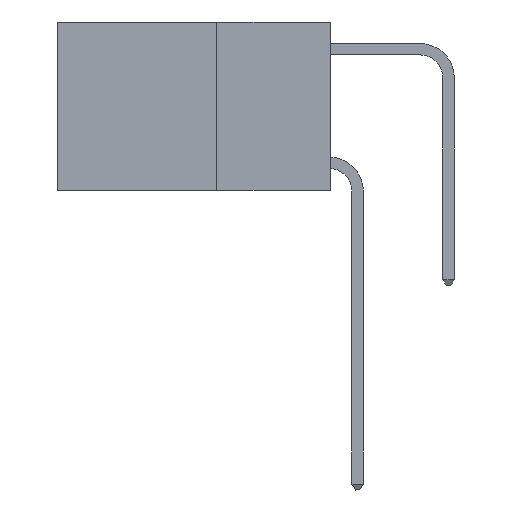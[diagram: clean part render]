
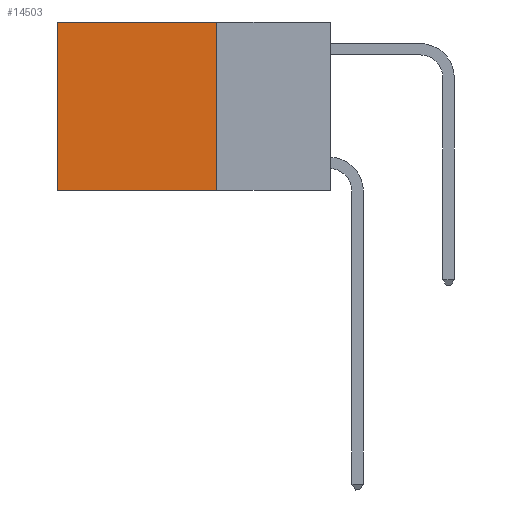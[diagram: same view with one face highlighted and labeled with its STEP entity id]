
A CAD part, left-side view. The second image highlights one B-rep face of the part: STEP entity #14503.
In plain terms, the highlighted planar face has unit normal (-1, 0, 0).
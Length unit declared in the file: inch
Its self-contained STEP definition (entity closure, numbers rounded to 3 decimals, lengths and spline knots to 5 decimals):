
#30 = VECTOR ( 'NONE', #21371, 39.37008 ) ;
#806 = LINE ( 'NONE', #18904, #30 ) ;
#2527 = LINE ( 'NONE', #7097, #28659 ) ;
#2807 = CARTESIAN_POINT ( 'NONE',  ( 0.2625, 0.25, 0. ) ) ;
#4504 = CARTESIAN_POINT ( 'NONE',  ( 0.2625, 0.6, 0. ) ) ;
#5294 = DIRECTION ( 'NONE',  ( 0., 0., -1. ) ) ;
#5310 = CARTESIAN_POINT ( 'NONE',  ( 0.2625, 0.6, -0.37 ) ) ;
#5566 = CARTESIAN_POINT ( 'NONE',  ( 0.2625, 0.6, 0. ) ) ;
#7097 = CARTESIAN_POINT ( 'NONE',  ( 0.2625, 0.25, -0.37 ) ) ;
#7656 = CARTESIAN_POINT ( 'NONE',  ( 0.2625, 0.25, -0.37 ) ) ;
#8354 = EDGE_LOOP ( 'NONE', ( #23947, #12407, #8984, #13830 ) ) ;
#8430 = FACE_OUTER_BOUND ( 'NONE', #8354, .T. ) ;
#8984 = ORIENTED_EDGE ( 'NONE', *, *, #10414, .F. ) ;
#9046 = DIRECTION ( 'NONE',  ( 0., 1., 0. ) ) ;
#9617 = EDGE_CURVE ( 'NONE', #18815, #29434, #30044, .T. ) ;
#10128 = PLANE ( 'NONE',  #31308 ) ;
#10414 = EDGE_CURVE ( 'NONE', #20979, #28552, #806, .T. ) ;
#11082 = VECTOR ( 'NONE', #9046, 39.37008 ) ;
#12407 = ORIENTED_EDGE ( 'NONE', *, *, #29080, .F. ) ;
#13830 = ORIENTED_EDGE ( 'NONE', *, *, #22159, .T. ) ;
#14503 = ADVANCED_FACE ( 'NONE', ( #8430 ), #10128, .F. ) ;
#17810 = VECTOR ( 'NONE', #27795, 39.37008 ) ;
#18815 = VERTEX_POINT ( 'NONE', #4504 ) ;
#18904 = CARTESIAN_POINT ( 'NONE',  ( 0.2625, 0.25, 0. ) ) ;
#20069 = DIRECTION ( 'NONE',  ( 1., 0., 0. ) ) ;
#20979 = VERTEX_POINT ( 'NONE', #23928 ) ;
#21342 = CARTESIAN_POINT ( 'NONE',  ( 0.2625, 0.25, 0. ) ) ;
#21371 = DIRECTION ( 'NONE',  ( 0., 0., -1. ) ) ;
#22159 = EDGE_CURVE ( 'NONE', #20979, #18815, #30990, .T. ) ;
#23928 = CARTESIAN_POINT ( 'NONE',  ( 0.2625, 0.25, 0. ) ) ;
#23947 = ORIENTED_EDGE ( 'NONE', *, *, #9617, .T. ) ;
#27795 = DIRECTION ( 'NONE',  ( 0., 0., -1. ) ) ;
#28552 = VERTEX_POINT ( 'NONE', #7656 ) ;
#28659 = VECTOR ( 'NONE', #31662, 39.37008 ) ;
#29080 = EDGE_CURVE ( 'NONE', #28552, #29434, #2527, .T. ) ;
#29434 = VERTEX_POINT ( 'NONE', #5310 ) ;
#30044 = LINE ( 'NONE', #5566, #17810 ) ;
#30990 = LINE ( 'NONE', #21342, #11082 ) ;
#31308 = AXIS2_PLACEMENT_3D ( 'NONE', #2807, #20069, #5294 ) ;
#31662 = DIRECTION ( 'NONE',  ( 0., 1., 0. ) ) ;
